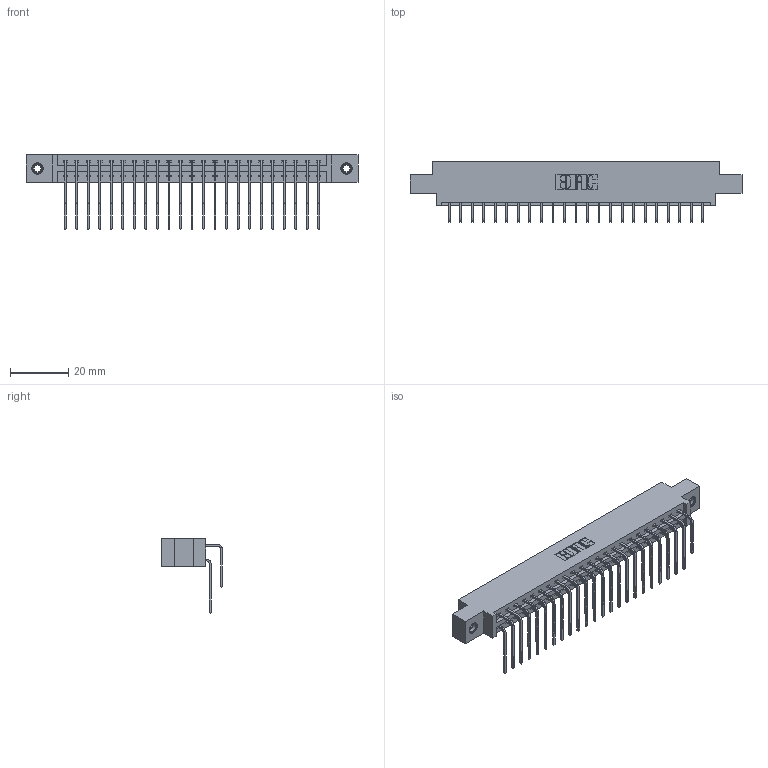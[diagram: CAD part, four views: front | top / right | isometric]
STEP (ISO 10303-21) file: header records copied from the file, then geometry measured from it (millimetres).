
FILE_DESCRIPTION (( 'STEP AP203' ), '1' );
FILE_NAME ('387-046-559-807.STEP', '2019-10-18T08:41:22', ( '' ), ( '' ), 'SwSTEP 2.0', 'SolidWorks 2016', '' );
FILE_SCHEMA (( 'CONFIG_CONTROL_DESIGN' ));
Length unit declared in the file: inch
Products named in the file (5): 337 Part_0.170 Offset - 0.156 Dia-TI; 387-046-559-807; 345-292-001_559 Tail - 2; 345-250-001_345-250-005-103; 345-292-001_558 559 Tail - 1
Assembly tree (49 placements, depth 2):
  387-046-559-807
    337 Part_0.170 Offset - 0.156 Dia-TI
    345-292-001_558 559 Tail - 1  x23
    345-292-001_559 Tail - 2  x23
    345-250-001_345-250-005-103  x2
Bounding box: 114.15 x 20.9 x 25.53 mm (x, y, z)
Volume: 11911.2 mm3; surface area: 14757.3 mm2
Topology: 49 solids, 49 shells, 2754 faces, 8141 edges, 5358 vertices
Faces by surface type: plane 1946, cylinder 792, cone 12, torus 4
Entity records: 23392 total; most frequent: CARTESIAN_POINT 3984, ORIENTED_EDGE 3862, DIRECTION 3437, EDGE_CURVE 1931, VECTOR 1743, LINE 1743, VERTEX_POINT 1280, AXIS2_PLACEMENT_3D 847
